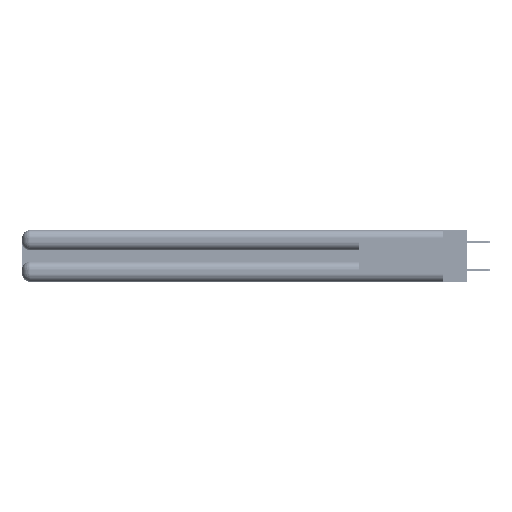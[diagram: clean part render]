
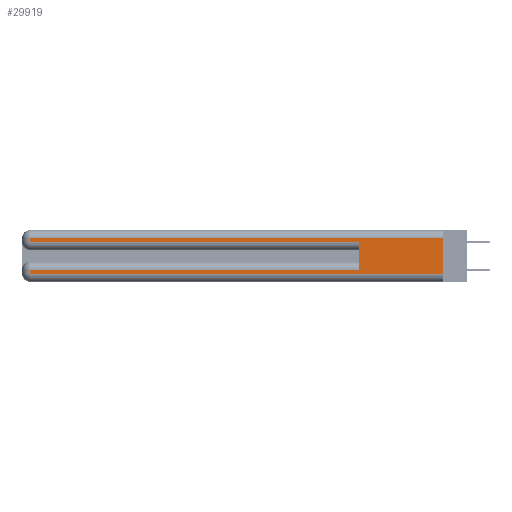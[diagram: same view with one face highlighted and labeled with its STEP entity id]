
A CAD part, left-side view. The second image highlights one B-rep face of the part: STEP entity #29919.
In plain terms, the highlighted planar face has unit normal (-1, 0, 0).
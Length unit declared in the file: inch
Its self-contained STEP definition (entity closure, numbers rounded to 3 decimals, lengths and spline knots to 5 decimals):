
#247 = ORIENTED_EDGE ( 'NONE', *, *, #53529, .F. ) ;
#2826 = CARTESIAN_POINT ( 'NONE',  ( 0., 0.6, 0.285 ) ) ;
#2835 = DIRECTION ( 'NONE',  ( 0., 0., -1. ) ) ;
#3436 = CARTESIAN_POINT ( 'NONE',  ( 0., 2.94, 0.37 ) ) ;
#4026 = CARTESIAN_POINT ( 'NONE',  ( 0., 0., 0.085 ) ) ;
#4994 = EDGE_CURVE ( 'NONE', #9561, #44716, #23441, .T. ) ;
#5922 = AXIS2_PLACEMENT_3D ( 'NONE', #14903, #44497, #40801 ) ;
#6407 = VECTOR ( 'NONE', #2835, 39.37008 ) ;
#6508 = LINE ( 'NONE', #3436, #27627 ) ;
#6620 = LINE ( 'NONE', #53336, #16527 ) ;
#7984 = EDGE_CURVE ( 'NONE', #28550, #53455, #40267, .T. ) ;
#7991 = CARTESIAN_POINT ( 'NONE',  ( 0., 2.94, 0.37 ) ) ;
#9561 = VERTEX_POINT ( 'NONE', #30408 ) ;
#11805 = EDGE_CURVE ( 'NONE', #29333, #33839, #21790, .T. ) ;
#13427 = EDGE_CURVE ( 'NONE', #33839, #25910, #46027, .T. ) ;
#13504 = VECTOR ( 'NONE', #38094, 39.37008 ) ;
#14141 = LINE ( 'NONE', #4026, #13504 ) ;
#14903 = CARTESIAN_POINT ( 'NONE',  ( 0., 0., 0.37 ) ) ;
#16527 = VECTOR ( 'NONE', #20171, 39.37008 ) ;
#17140 = CARTESIAN_POINT ( 'NONE',  ( 0., 2.94, 0.06 ) ) ;
#19086 = CARTESIAN_POINT ( 'NONE',  ( 0., 0., 0.06 ) ) ;
#19278 = CARTESIAN_POINT ( 'NONE',  ( 0., 0., 0.37 ) ) ;
#20171 = DIRECTION ( 'NONE',  ( 0., -1., 0. ) ) ;
#21470 = DIRECTION ( 'NONE',  ( 0., 1., 0. ) ) ;
#21790 = LINE ( 'NONE', #7991, #48784 ) ;
#21821 = ORIENTED_EDGE ( 'NONE', *, *, #7984, .T. ) ;
#22109 = VECTOR ( 'NONE', #53513, 39.37008 ) ;
#22309 = VECTOR ( 'NONE', #48900, 39.37008 ) ;
#23441 = LINE ( 'NONE', #37075, #22109 ) ;
#24001 = ORIENTED_EDGE ( 'NONE', *, *, #48880, .T. ) ;
#25831 = VECTOR ( 'NONE', #21470, 39.37008 ) ;
#25910 = VERTEX_POINT ( 'NONE', #40751 ) ;
#27013 = CARTESIAN_POINT ( 'NONE',  ( 0., 2.94, 0.31 ) ) ;
#27627 = VECTOR ( 'NONE', #32932, 39.37008 ) ;
#28313 = ORIENTED_EDGE ( 'NONE', *, *, #46574, .T. ) ;
#28550 = VERTEX_POINT ( 'NONE', #44759 ) ;
#29333 = VERTEX_POINT ( 'NONE', #45666 ) ;
#29919 = ADVANCED_FACE ( 'NONE', ( #36868 ), #40078, .F. ) ;
#30069 = ORIENTED_EDGE ( 'NONE', *, *, #13427, .T. ) ;
#30408 = CARTESIAN_POINT ( 'NONE',  ( 0., 0.6, 0.085 ) ) ;
#32115 = LINE ( 'NONE', #19278, #6407 ) ;
#32932 = DIRECTION ( 'NONE',  ( 0., 0., -1. ) ) ;
#33839 = VERTEX_POINT ( 'NONE', #17140 ) ;
#36868 = FACE_OUTER_BOUND ( 'NONE', #37724, .T. ) ;
#37075 = CARTESIAN_POINT ( 'NONE',  ( 0., 0.6, 0.145 ) ) ;
#37105 = CARTESIAN_POINT ( 'NONE',  ( 0., 2.94, 0.285 ) ) ;
#37724 = EDGE_LOOP ( 'NONE', ( #247, #21821, #38210, #28313, #50165, #24001, #41883, #30069 ) ) ;
#38094 = DIRECTION ( 'NONE',  ( 0., 1., 0. ) ) ;
#38210 = ORIENTED_EDGE ( 'NONE', *, *, #47616, .T. ) ;
#40078 = PLANE ( 'NONE',  #5922 ) ;
#40267 = LINE ( 'NONE', #51291, #25831 ) ;
#40751 = CARTESIAN_POINT ( 'NONE',  ( 0., 0., 0.06 ) ) ;
#40801 = DIRECTION ( 'NONE',  ( 0., 0., -1. ) ) ;
#41883 = ORIENTED_EDGE ( 'NONE', *, *, #11805, .T. ) ;
#44497 = DIRECTION ( 'NONE',  ( 1., 0., 0. ) ) ;
#44716 = VERTEX_POINT ( 'NONE', #2826 ) ;
#44759 = CARTESIAN_POINT ( 'NONE',  ( 0., 0., 0.31 ) ) ;
#45666 = CARTESIAN_POINT ( 'NONE',  ( 0., 2.94, 0.085 ) ) ;
#46027 = LINE ( 'NONE', #19086, #22309 ) ;
#46574 = EDGE_CURVE ( 'NONE', #50836, #44716, #6620, .T. ) ;
#47616 = EDGE_CURVE ( 'NONE', #53455, #50836, #6508, .T. ) ;
#48784 = VECTOR ( 'NONE', #54046, 39.37008 ) ;
#48880 = EDGE_CURVE ( 'NONE', #9561, #29333, #14141, .T. ) ;
#48900 = DIRECTION ( 'NONE',  ( 0., -1., 0. ) ) ;
#50165 = ORIENTED_EDGE ( 'NONE', *, *, #4994, .F. ) ;
#50836 = VERTEX_POINT ( 'NONE', #37105 ) ;
#51291 = CARTESIAN_POINT ( 'NONE',  ( 0., 0., 0.31 ) ) ;
#53336 = CARTESIAN_POINT ( 'NONE',  ( 0., 0., 0.285 ) ) ;
#53455 = VERTEX_POINT ( 'NONE', #27013 ) ;
#53513 = DIRECTION ( 'NONE',  ( 0., 0., 1. ) ) ;
#53529 = EDGE_CURVE ( 'NONE', #28550, #25910, #32115, .T. ) ;
#54046 = DIRECTION ( 'NONE',  ( 0., 0., -1. ) ) ;
